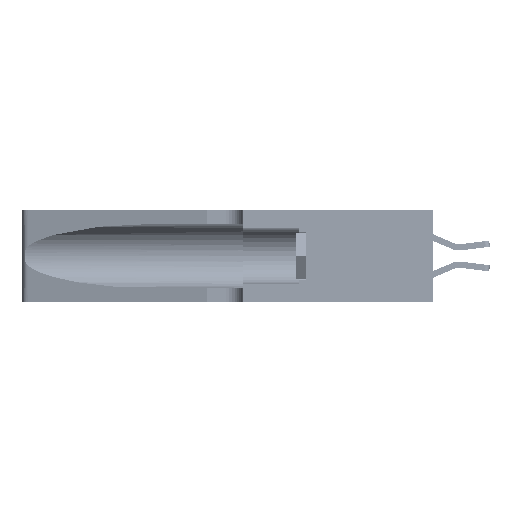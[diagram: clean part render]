
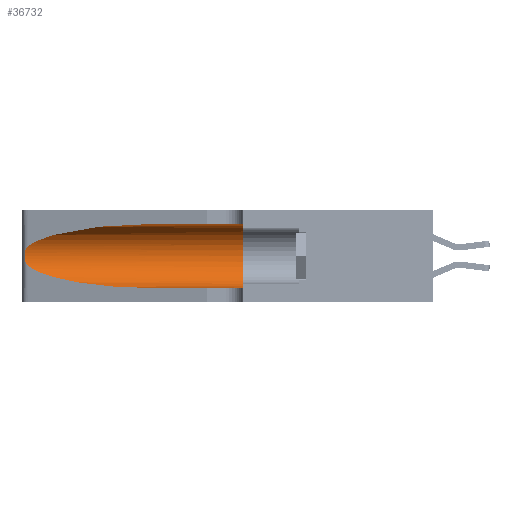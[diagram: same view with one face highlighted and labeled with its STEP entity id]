
A CAD part, left-side view. The second image highlights one B-rep face of the part: STEP entity #36732.
In plain terms, the highlighted cylindrical face has radius 3.308 mm (diameter 6.617 mm), a partial arc.
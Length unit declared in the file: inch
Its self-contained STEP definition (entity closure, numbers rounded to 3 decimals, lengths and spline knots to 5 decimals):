
#156 = CARTESIAN_POINT ( 'NONE',  ( 0.1305, 0.35, 0.185 ) ) ;
#2432 = DIRECTION ( 'NONE',  ( 0., 0., -1. ) ) ;
#3797 = VERTEX_POINT ( 'NONE', #9362 ) ;
#3934 = DIRECTION ( 'NONE',  ( 0., 0., 1. ) ) ;
#3977 = CARTESIAN_POINT ( 'NONE',  ( 0.2373, 1.15595, 0.28018 ) ) ;
#3983 = CARTESIAN_POINT ( 'NONE',  ( 0.1305, 0.35, 0.05475 ) ) ;
#4732 =( BOUNDED_CURVE ( )  B_SPLINE_CURVE ( 3, ( #31065, #41700, #34677, #12852 ),
 .UNSPECIFIED., .F., .F. ) 
 B_SPLINE_CURVE_WITH_KNOTS ( ( 4, 4 ),
 ( 3.44316, 4.71239 ),
 .UNSPECIFIED. ) 
 CURVE ( )  GEOMETRIC_REPRESENTATION_ITEM ( )  RATIONAL_B_SPLINE_CURVE ( ( 1., 0.87, 0.87, 1. ) ) 
 REPRESENTATION_ITEM ( '' )  );
#5105 = LINE ( 'NONE', #18232, #25871 ) ;
#7122 = CARTESIAN_POINT ( 'NONE',  ( 0.25787, 1.23484, 0.2124 ) ) ;
#7246 = DIRECTION ( 'NONE',  ( 0., -1., 0. ) ) ;
#7390 = DIRECTION ( 'NONE',  ( 0., -1., 0. ) ) ;
#7730 = EDGE_LOOP ( 'NONE', ( #25355, #31662, #23673, #33109, #40727, #27000 ) ) ;
#7737 = CYLINDRICAL_SURFACE ( 'NONE', #11096, 0.13025 ) ;
#7754 = CARTESIAN_POINT ( 'NONE',  ( 0.1305, 0.35, 0.31525 ) ) ;
#7954 = LINE ( 'NONE', #25719, #45459 ) ;
#9362 = CARTESIAN_POINT ( 'NONE',  ( 0.25487, 1.22718, 0.22369 ) ) ;
#9961 = CIRCLE ( 'NONE', #21574, 0.13025 ) ;
#10853 = CARTESIAN_POINT ( 'NONE',  ( 0.26018, 1.23835, 0.19895 ) ) ;
#11096 = AXIS2_PLACEMENT_3D ( 'NONE', #13543, #42512, #2432 ) ;
#12434 = VERTEX_POINT ( 'NONE', #3983 ) ;
#12852 = CARTESIAN_POINT ( 'NONE',  ( 0.1305, 0.72297, 0.05475 ) ) ;
#13276 = VERTEX_POINT ( 'NONE', #41401 ) ;
#13543 = CARTESIAN_POINT ( 'NONE',  ( 0.1305, 1.61858, 0.185 ) ) ;
#14569 = CARTESIAN_POINT ( 'NONE',  ( 0.26075, 1.23896, 0.178 ) ) ;
#14860 =( BOUNDED_CURVE ( )  B_SPLINE_CURVE ( 3, ( #40372, #15047, #3977, #29721 ),
 .UNSPECIFIED., .F., .F. ) 
 B_SPLINE_CURVE_WITH_KNOTS ( ( 4, 4 ),
 ( 1.5708, 2.84003 ),
 .UNSPECIFIED. ) 
 CURVE ( )  GEOMETRIC_REPRESENTATION_ITEM ( )  RATIONAL_B_SPLINE_CURVE ( ( 1., 0.87, 0.87, 1. ) ) 
 REPRESENTATION_ITEM ( '' )  );
#15047 = CARTESIAN_POINT ( 'NONE',  ( 0.18966, 0.96281, 0.31525 ) ) ;
#16630 = CARTESIAN_POINT ( 'NONE',  ( 0.25487, 1.22718, 0.14631 ) ) ;
#18232 = CARTESIAN_POINT ( 'NONE',  ( 0.1305, 1.61858, 0.31525 ) ) ;
#18272 = CARTESIAN_POINT ( 'NONE',  ( 0.25856, 1.23593, 0.16098 ) ) ;
#20641 = EDGE_CURVE ( 'NONE', #35998, #13276, #4732, .T. ) ;
#21574 = AXIS2_PLACEMENT_3D ( 'NONE', #156, #26020, #3934 ) ;
#21624 = CARTESIAN_POINT ( 'NONE',  ( 0.25487, 1.22718, 0.22369 ) ) ;
#21945 = CARTESIAN_POINT ( 'NONE',  ( 0.25639, 1.23186, 0.15144 ) ) ;
#23673 = ORIENTED_EDGE ( 'NONE', *, *, #20641, .T. ) ;
#25355 = ORIENTED_EDGE ( 'NONE', *, *, #43127, .T. ) ;
#25616 = CARTESIAN_POINT ( 'NONE',  ( 0.25487, 1.22718, 0.14631 ) ) ;
#25719 = CARTESIAN_POINT ( 'NONE',  ( 0.1305, 1.61858, 0.05475 ) ) ;
#25871 = VECTOR ( 'NONE', #7246, 39.37008 ) ;
#25984 = EDGE_CURVE ( 'NONE', #44855, #12434, #9961, .T. ) ;
#26020 = DIRECTION ( 'NONE',  ( 0., 1., 0. ) ) ;
#27000 = ORIENTED_EDGE ( 'NONE', *, *, #33346, .F. ) ;
#28413 = FACE_OUTER_BOUND ( 'NONE', #7730, .T. ) ;
#28478 = EDGE_CURVE ( 'NONE', #3797, #35998, #35263, .T. ) ;
#29093 = CARTESIAN_POINT ( 'NONE',  ( 0.25639, 1.23184, 0.21858 ) ) ;
#29171 = EDGE_CURVE ( 'NONE', #13276, #12434, #7954, .T. ) ;
#29721 = CARTESIAN_POINT ( 'NONE',  ( 0.25487, 1.22718, 0.22369 ) ) ;
#31065 = CARTESIAN_POINT ( 'NONE',  ( 0.25487, 1.22718, 0.14631 ) ) ;
#31662 = ORIENTED_EDGE ( 'NONE', *, *, #28478, .T. ) ;
#32750 = CARTESIAN_POINT ( 'NONE',  ( 0.25854, 1.2359, 0.20912 ) ) ;
#33109 = ORIENTED_EDGE ( 'NONE', *, *, #29171, .T. ) ;
#33346 = EDGE_CURVE ( 'NONE', #42140, #44855, #5105, .T. ) ;
#34677 = CARTESIAN_POINT ( 'NONE',  ( 0.18966, 0.96281, 0.05475 ) ) ;
#35263 = B_SPLINE_CURVE_WITH_KNOTS ( 'NONE', 3,
 ( #21624, #39758, #29093, #7122, #32750, #10853, #36334, #14569, #39911, #18272, #43517, #21945, #47157, #25616 ),
 .UNSPECIFIED., .F., .F.,
 ( 4, 2, 2, 2, 2, 2, 4 ),
 ( 0., 0.00027, 0.00053, 0.00107, 0.0016, 0.00187, 0.00214 ),
 .UNSPECIFIED. ) ;
#35998 = VERTEX_POINT ( 'NONE', #16630 ) ;
#36334 = CARTESIAN_POINT ( 'NONE',  ( 0.26075, 1.23896, 0.19203 ) ) ;
#36732 = ADVANCED_FACE ( 'NONE', ( #28413 ), #7737, .F. ) ;
#39758 = CARTESIAN_POINT ( 'NONE',  ( 0.25555, 1.22994, 0.2215 ) ) ;
#39911 = CARTESIAN_POINT ( 'NONE',  ( 0.26017, 1.23833, 0.17102 ) ) ;
#40372 = CARTESIAN_POINT ( 'NONE',  ( 0.1305, 0.72297, 0.31525 ) ) ;
#40727 = ORIENTED_EDGE ( 'NONE', *, *, #25984, .F. ) ;
#41401 = CARTESIAN_POINT ( 'NONE',  ( 0.1305, 0.72297, 0.05475 ) ) ;
#41700 = CARTESIAN_POINT ( 'NONE',  ( 0.2373, 1.15595, 0.08982 ) ) ;
#42140 = VERTEX_POINT ( 'NONE', #45482 ) ;
#42512 = DIRECTION ( 'NONE',  ( 0., -1., 0. ) ) ;
#43127 = EDGE_CURVE ( 'NONE', #42140, #3797, #14860, .T. ) ;
#43517 = CARTESIAN_POINT ( 'NONE',  ( 0.25789, 1.23486, 0.15765 ) ) ;
#44855 = VERTEX_POINT ( 'NONE', #7754 ) ;
#45459 = VECTOR ( 'NONE', #7390, 39.37008 ) ;
#45482 = CARTESIAN_POINT ( 'NONE',  ( 0.1305, 0.72297, 0.31525 ) ) ;
#47157 = CARTESIAN_POINT ( 'NONE',  ( 0.25555, 1.22993, 0.14849 ) ) ;
